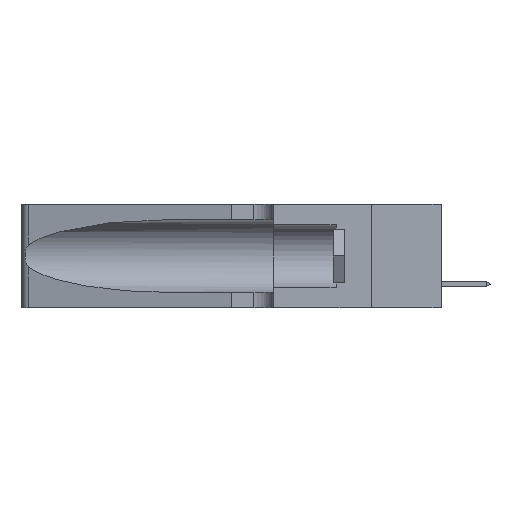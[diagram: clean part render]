
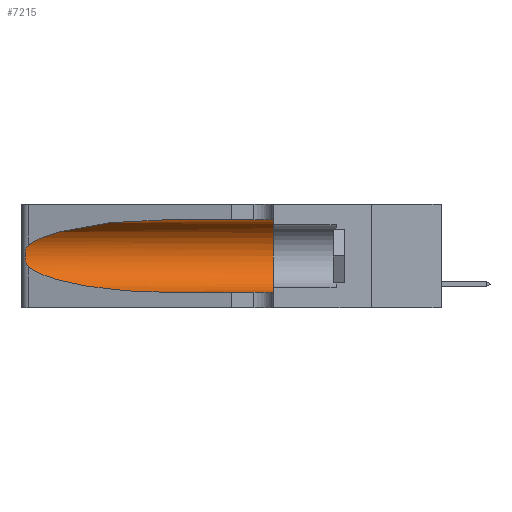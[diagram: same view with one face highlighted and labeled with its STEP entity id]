
A CAD part, left-side view. The second image highlights one B-rep face of the part: STEP entity #7215.
In plain terms, the highlighted cylindrical face has radius 3.308 mm (diameter 6.617 mm), a partial arc.
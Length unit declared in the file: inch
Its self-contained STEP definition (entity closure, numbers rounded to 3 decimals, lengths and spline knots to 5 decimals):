
#889 = CARTESIAN_POINT ( 'NONE',  ( 0.18966, 0.96281, 0.05475 ) ) ;
#1084 = CARTESIAN_POINT ( 'NONE',  ( 0.25487, 1.22718, 0.22369 ) ) ;
#2836 = CARTESIAN_POINT ( 'NONE',  ( 0.25789, 1.23486, 0.15765 ) ) ;
#3107 =( BOUNDED_CURVE ( )  B_SPLINE_CURVE ( 3, ( #23107, #15771, #889, #19262 ),
 .UNSPECIFIED., .F., .F. ) 
 B_SPLINE_CURVE_WITH_KNOTS ( ( 4, 4 ),
 ( 3.44316, 4.71239 ),
 .UNSPECIFIED. ) 
 CURVE ( )  GEOMETRIC_REPRESENTATION_ITEM ( )  RATIONAL_B_SPLINE_CURVE ( ( 1., 0.87, 0.87, 1. ) ) 
 REPRESENTATION_ITEM ( '' )  );
#3286 = ORIENTED_EDGE ( 'NONE', *, *, #20651, .T. ) ;
#3709 = VERTEX_POINT ( 'NONE', #1084 ) ;
#4352 = ORIENTED_EDGE ( 'NONE', *, *, #19261, .T. ) ;
#6277 = CARTESIAN_POINT ( 'NONE',  ( 0.18966, 0.96281, 0.31525 ) ) ;
#7215 = ADVANCED_FACE ( 'NONE', ( #42860 ), #7220, .F. ) ;
#7220 = CYLINDRICAL_SURFACE ( 'NONE', #13976, 0.13025 ) ;
#7307 = VECTOR ( 'NONE', #18504, 39.37008 ) ;
#7420 = CARTESIAN_POINT ( 'NONE',  ( 0.1305, 1.61858, 0.31525 ) ) ;
#7874 = DIRECTION ( 'NONE',  ( 0., -1., 0. ) ) ;
#9301 = CARTESIAN_POINT ( 'NONE',  ( 0.1305, 0.35, 0.31525 ) ) ;
#9674 = EDGE_CURVE ( 'NONE', #17354, #3709, #31166, .T. ) ;
#11874 = LINE ( 'NONE', #38212, #48834 ) ;
#12363 = CIRCLE ( 'NONE', #39680, 0.13025 ) ;
#13053 = VERTEX_POINT ( 'NONE', #28717 ) ;
#13976 = AXIS2_PLACEMENT_3D ( 'NONE', #25937, #7874, #15266 ) ;
#14556 = CARTESIAN_POINT ( 'NONE',  ( 0.26075, 1.23896, 0.178 ) ) ;
#15020 = ORIENTED_EDGE ( 'NONE', *, *, #26701, .F. ) ;
#15266 = DIRECTION ( 'NONE',  ( 0., 0., -1. ) ) ;
#15771 = CARTESIAN_POINT ( 'NONE',  ( 0.2373, 1.15595, 0.08982 ) ) ;
#15913 = EDGE_CURVE ( 'NONE', #13053, #29918, #3107, .T. ) ;
#16423 = CARTESIAN_POINT ( 'NONE',  ( 0.25487, 1.22718, 0.22369 ) ) ;
#17354 = VERTEX_POINT ( 'NONE', #38440 ) ;
#17477 = LINE ( 'NONE', #7420, #7307 ) ;
#18504 = DIRECTION ( 'NONE',  ( 0., -1., 0. ) ) ;
#19261 = EDGE_CURVE ( 'NONE', #29918, #40183, #11874, .T. ) ;
#19262 = CARTESIAN_POINT ( 'NONE',  ( 0.1305, 0.72297, 0.05475 ) ) ;
#20234 = CARTESIAN_POINT ( 'NONE',  ( 0.25555, 1.22994, 0.2215 ) ) ;
#20306 = ORIENTED_EDGE ( 'NONE', *, *, #15913, .T. ) ;
#20651 = EDGE_CURVE ( 'NONE', #3709, #13053, #26052, .T. ) ;
#22076 = CARTESIAN_POINT ( 'NONE',  ( 0.25787, 1.23484, 0.2124 ) ) ;
#22634 = ORIENTED_EDGE ( 'NONE', *, *, #35231, .F. ) ;
#23107 = CARTESIAN_POINT ( 'NONE',  ( 0.25487, 1.22718, 0.14631 ) ) ;
#25492 = CARTESIAN_POINT ( 'NONE',  ( 0.1305, 0.72297, 0.31525 ) ) ;
#25711 = CARTESIAN_POINT ( 'NONE',  ( 0.25487, 1.22718, 0.14631 ) ) ;
#25937 = CARTESIAN_POINT ( 'NONE',  ( 0.1305, 1.61858, 0.185 ) ) ;
#26052 = B_SPLINE_CURVE_WITH_KNOTS ( 'NONE', 3,
 ( #16423, #20234, #48670, #22076, #48336, #33185, #48183, #14556, #36802, #40479, #2836, #33033, #32852, #25711 ),
 .UNSPECIFIED., .F., .F.,
 ( 4, 2, 2, 2, 2, 2, 4 ),
 ( 0., 0.00027, 0.00053, 0.00107, 0.0016, 0.00187, 0.00214 ),
 .UNSPECIFIED. ) ;
#26701 = EDGE_CURVE ( 'NONE', #17354, #28207, #17477, .T. ) ;
#28001 = DIRECTION ( 'NONE',  ( 0., 0., 1. ) ) ;
#28207 = VERTEX_POINT ( 'NONE', #9301 ) ;
#28717 = CARTESIAN_POINT ( 'NONE',  ( 0.25487, 1.22718, 0.14631 ) ) ;
#28942 = CARTESIAN_POINT ( 'NONE',  ( 0.25487, 1.22718, 0.22369 ) ) ;
#29918 = VERTEX_POINT ( 'NONE', #36377 ) ;
#30819 = EDGE_LOOP ( 'NONE', ( #45367, #3286, #20306, #4352, #22634, #15020 ) ) ;
#31166 =( BOUNDED_CURVE ( )  B_SPLINE_CURVE ( 3, ( #25492, #6277, #33134, #28942 ),
 .UNSPECIFIED., .F., .T. ) 
 B_SPLINE_CURVE_WITH_KNOTS ( ( 4, 4 ),
 ( 1.5708, 2.84003 ),
 .UNSPECIFIED. ) 
 CURVE ( )  GEOMETRIC_REPRESENTATION_ITEM ( )  RATIONAL_B_SPLINE_CURVE ( ( 1., 0.87, 0.87, 1. ) ) 
 REPRESENTATION_ITEM ( '' )  );
#32852 = CARTESIAN_POINT ( 'NONE',  ( 0.25555, 1.22993, 0.14849 ) ) ;
#33033 = CARTESIAN_POINT ( 'NONE',  ( 0.25639, 1.23186, 0.15144 ) ) ;
#33134 = CARTESIAN_POINT ( 'NONE',  ( 0.2373, 1.15595, 0.28018 ) ) ;
#33185 = CARTESIAN_POINT ( 'NONE',  ( 0.26018, 1.23835, 0.19895 ) ) ;
#35231 = EDGE_CURVE ( 'NONE', #28207, #40183, #12363, .T. ) ;
#36377 = CARTESIAN_POINT ( 'NONE',  ( 0.1305, 0.72297, 0.05475 ) ) ;
#36802 = CARTESIAN_POINT ( 'NONE',  ( 0.26017, 1.23833, 0.17102 ) ) ;
#38212 = CARTESIAN_POINT ( 'NONE',  ( 0.1305, 1.61858, 0.05475 ) ) ;
#38440 = CARTESIAN_POINT ( 'NONE',  ( 0.1305, 0.72297, 0.31525 ) ) ;
#38510 = CARTESIAN_POINT ( 'NONE',  ( 0.1305, 0.35, 0.185 ) ) ;
#38546 = DIRECTION ( 'NONE',  ( 0., -1., 0. ) ) ;
#39680 = AXIS2_PLACEMENT_3D ( 'NONE', #38510, #47348, #28001 ) ;
#40183 = VERTEX_POINT ( 'NONE', #45240 ) ;
#40479 = CARTESIAN_POINT ( 'NONE',  ( 0.25856, 1.23593, 0.16098 ) ) ;
#42860 = FACE_OUTER_BOUND ( 'NONE', #30819, .T. ) ;
#45240 = CARTESIAN_POINT ( 'NONE',  ( 0.1305, 0.35, 0.05475 ) ) ;
#45367 = ORIENTED_EDGE ( 'NONE', *, *, #9674, .T. ) ;
#47348 = DIRECTION ( 'NONE',  ( 0., 1., 0. ) ) ;
#48183 = CARTESIAN_POINT ( 'NONE',  ( 0.26075, 1.23896, 0.19203 ) ) ;
#48336 = CARTESIAN_POINT ( 'NONE',  ( 0.25854, 1.2359, 0.20912 ) ) ;
#48670 = CARTESIAN_POINT ( 'NONE',  ( 0.25639, 1.23184, 0.21858 ) ) ;
#48834 = VECTOR ( 'NONE', #38546, 39.37008 ) ;
